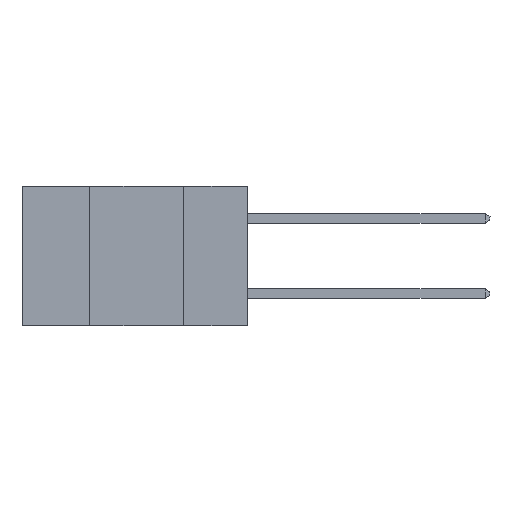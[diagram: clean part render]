
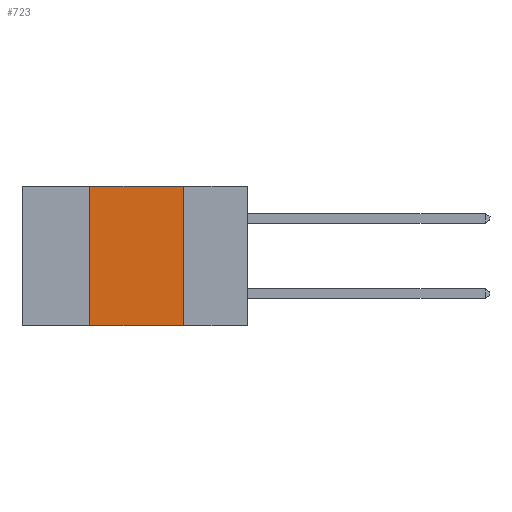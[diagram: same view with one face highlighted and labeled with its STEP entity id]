
A CAD part, left-side view. The second image highlights one B-rep face of the part: STEP entity #723.
In plain terms, the highlighted planar face has unit normal (-1, 0, 0).
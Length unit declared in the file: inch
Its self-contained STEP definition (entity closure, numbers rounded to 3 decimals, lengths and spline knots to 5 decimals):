
#335 = VERTEX_POINT ( 'NONE', #4613 ) ;
#723 = ADVANCED_FACE ( 'NONE', ( #5060 ), #5808, .F. ) ;
#769 = DIRECTION ( 'NONE',  ( 0., 0., -1. ) ) ;
#773 = CARTESIAN_POINT ( 'NONE',  ( 0., 0.6, 0. ) ) ;
#1069 = AXIS2_PLACEMENT_3D ( 'NONE', #773, #4451, #3609 ) ;
#2171 = DIRECTION ( 'NONE',  ( 0., 0., 1. ) ) ;
#2179 = VERTEX_POINT ( 'NONE', #8522 ) ;
#2335 = VERTEX_POINT ( 'NONE', #3075 ) ;
#2776 = DIRECTION ( 'NONE',  ( 0., -1., 0. ) ) ;
#2879 = CARTESIAN_POINT ( 'NONE',  ( 0., 0.42, -0.37 ) ) ;
#2911 = CARTESIAN_POINT ( 'NONE',  ( 0., 0.17, -0.37 ) ) ;
#3075 = CARTESIAN_POINT ( 'NONE',  ( 0., 0.17, 0. ) ) ;
#3132 = ORIENTED_EDGE ( 'NONE', *, *, #7980, .F. ) ;
#3269 = LINE ( 'NONE', #7430, #5738 ) ;
#3437 = VECTOR ( 'NONE', #2171, 39.37008 ) ;
#3506 = EDGE_LOOP ( 'NONE', ( #3132, #7037, #6185, #6257 ) ) ;
#3549 = EDGE_CURVE ( 'NONE', #7554, #2179, #5062, .T. ) ;
#3609 = DIRECTION ( 'NONE',  ( 0., 0., -1. ) ) ;
#3820 = DIRECTION ( 'NONE',  ( 0., -1., 0. ) ) ;
#4347 = LINE ( 'NONE', #2911, #4883 ) ;
#4451 = DIRECTION ( 'NONE',  ( 1., 0., 0. ) ) ;
#4453 = CARTESIAN_POINT ( 'NONE',  ( 0., 0.42, -0.37 ) ) ;
#4613 = CARTESIAN_POINT ( 'NONE',  ( 0., 0.17, -0.37 ) ) ;
#4616 = EDGE_CURVE ( 'NONE', #7554, #335, #4972, .T. ) ;
#4883 = VECTOR ( 'NONE', #769, 39.37008 ) ;
#4972 = LINE ( 'NONE', #9111, #8572 ) ;
#5060 = FACE_OUTER_BOUND ( 'NONE', #3506, .T. ) ;
#5062 = LINE ( 'NONE', #4453, #3437 ) ;
#5738 = VECTOR ( 'NONE', #3820, 39.37008 ) ;
#5808 = PLANE ( 'NONE',  #1069 ) ;
#6185 = ORIENTED_EDGE ( 'NONE', *, *, #3549, .F. ) ;
#6257 = ORIENTED_EDGE ( 'NONE', *, *, #4616, .T. ) ;
#6717 = EDGE_CURVE ( 'NONE', #2179, #2335, #3269, .T. ) ;
#7037 = ORIENTED_EDGE ( 'NONE', *, *, #6717, .F. ) ;
#7430 = CARTESIAN_POINT ( 'NONE',  ( 0., 0.6, 0. ) ) ;
#7554 = VERTEX_POINT ( 'NONE', #2879 ) ;
#7980 = EDGE_CURVE ( 'NONE', #2335, #335, #4347, .T. ) ;
#8522 = CARTESIAN_POINT ( 'NONE',  ( 0., 0.42, 0. ) ) ;
#8572 = VECTOR ( 'NONE', #2776, 39.37008 ) ;
#9111 = CARTESIAN_POINT ( 'NONE',  ( 0., 0.6, -0.37 ) ) ;
